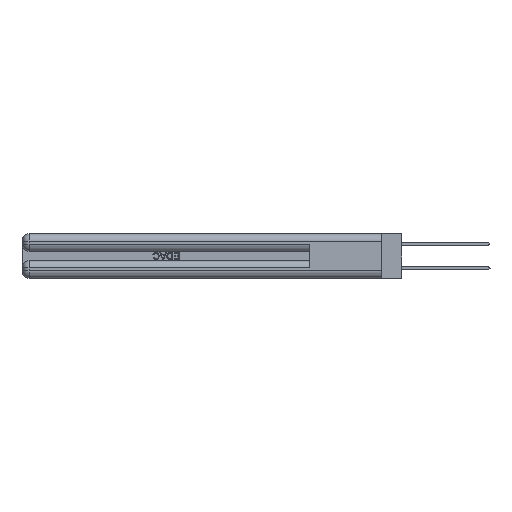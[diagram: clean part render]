
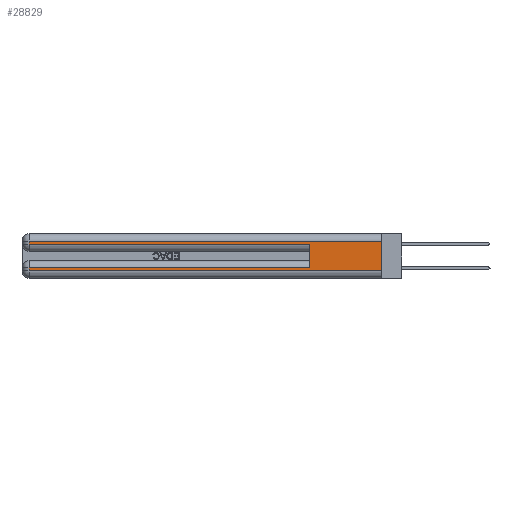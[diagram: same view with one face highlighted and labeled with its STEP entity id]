
A CAD part, left-side view. The second image highlights one B-rep face of the part: STEP entity #28829.
In plain terms, the highlighted planar face has unit normal (-1, 0, 0).
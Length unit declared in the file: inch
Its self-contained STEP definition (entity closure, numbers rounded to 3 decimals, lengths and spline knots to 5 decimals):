
#84 = EDGE_LOOP ( 'NONE', ( #25162, #44697, #18484, #17534, #12788, #21124, #45111, #26878 ) ) ;
#204 = LINE ( 'NONE', #20221, #9230 ) ;
#442 = CARTESIAN_POINT ( 'NONE',  ( 0., 2.94, 0.37 ) ) ;
#606 = LINE ( 'NONE', #25662, #39991 ) ;
#1106 = CARTESIAN_POINT ( 'NONE',  ( 0., 0., 0.285 ) ) ;
#1189 = DIRECTION ( 'NONE',  ( 0., -1., 0. ) ) ;
#2101 = DIRECTION ( 'NONE',  ( 0., 0., -1. ) ) ;
#2465 = LINE ( 'NONE', #12837, #32229 ) ;
#2803 = DIRECTION ( 'NONE',  ( 0., 0., -1. ) ) ;
#2838 = EDGE_CURVE ( 'NONE', #12835, #13054, #606, .T. ) ;
#3818 = AXIS2_PLACEMENT_3D ( 'NONE', #45466, #9768, #2101 ) ;
#4753 = DIRECTION ( 'NONE',  ( 0., -1., 0. ) ) ;
#5689 = VECTOR ( 'NONE', #1189, 39.37008 ) ;
#5760 = VERTEX_POINT ( 'NONE', #44814 ) ;
#6416 = DIRECTION ( 'NONE',  ( 0., 1., 0. ) ) ;
#9230 = VECTOR ( 'NONE', #2803, 39.37008 ) ;
#9733 = VECTOR ( 'NONE', #29216, 39.37008 ) ;
#9768 = DIRECTION ( 'NONE',  ( 1., 0., 0. ) ) ;
#10268 = EDGE_CURVE ( 'NONE', #5760, #13469, #204, .T. ) ;
#10463 = EDGE_CURVE ( 'NONE', #18079, #36989, #13769, .T. ) ;
#12788 = ORIENTED_EDGE ( 'NONE', *, *, #28244, .F. ) ;
#12835 = VERTEX_POINT ( 'NONE', #17748 ) ;
#12837 = CARTESIAN_POINT ( 'NONE',  ( 0., 0., 0.31 ) ) ;
#13054 = VERTEX_POINT ( 'NONE', #21293 ) ;
#13469 = VERTEX_POINT ( 'NONE', #37932 ) ;
#13769 = LINE ( 'NONE', #36397, #35679 ) ;
#14062 = LINE ( 'NONE', #40643, #5689 ) ;
#14242 = LINE ( 'NONE', #442, #9733 ) ;
#16396 = PLANE ( 'NONE',  #3818 ) ;
#16541 = EDGE_CURVE ( 'NONE', #13469, #19829, #45794, .T. ) ;
#16956 = EDGE_CURVE ( 'NONE', #18079, #5760, #2465, .T. ) ;
#17534 = ORIENTED_EDGE ( 'NONE', *, *, #16541, .T. ) ;
#17748 = CARTESIAN_POINT ( 'NONE',  ( 0., 0.6, 0.085 ) ) ;
#18079 = VERTEX_POINT ( 'NONE', #24294 ) ;
#18484 = ORIENTED_EDGE ( 'NONE', *, *, #10268, .T. ) ;
#19829 = VERTEX_POINT ( 'NONE', #42049 ) ;
#20221 = CARTESIAN_POINT ( 'NONE',  ( 0., 2.94, 0.37 ) ) ;
#21124 = ORIENTED_EDGE ( 'NONE', *, *, #2838, .T. ) ;
#21293 = CARTESIAN_POINT ( 'NONE',  ( 0., 2.94, 0.085 ) ) ;
#24294 = CARTESIAN_POINT ( 'NONE',  ( 0., 0., 0.31 ) ) ;
#24544 = EDGE_CURVE ( 'NONE', #13054, #43459, #14242, .T. ) ;
#25162 = ORIENTED_EDGE ( 'NONE', *, *, #10463, .F. ) ;
#25662 = CARTESIAN_POINT ( 'NONE',  ( 0., 0., 0.085 ) ) ;
#26263 = FACE_OUTER_BOUND ( 'NONE', #84, .T. ) ;
#26659 = VECTOR ( 'NONE', #4753, 39.37008 ) ;
#26878 = ORIENTED_EDGE ( 'NONE', *, *, #45808, .T. ) ;
#28244 = EDGE_CURVE ( 'NONE', #12835, #19829, #43758, .T. ) ;
#28829 = ADVANCED_FACE ( 'NONE', ( #26263 ), #16396, .F. ) ;
#29091 = CARTESIAN_POINT ( 'NONE',  ( 0., 2.94, 0.06 ) ) ;
#29216 = DIRECTION ( 'NONE',  ( 0., 0., -1. ) ) ;
#30127 = DIRECTION ( 'NONE',  ( 0., 0., 1. ) ) ;
#30285 = CARTESIAN_POINT ( 'NONE',  ( 0., 0.6, 0.145 ) ) ;
#30836 = VECTOR ( 'NONE', #30127, 39.37008 ) ;
#32229 = VECTOR ( 'NONE', #6416, 39.37008 ) ;
#35679 = VECTOR ( 'NONE', #36873, 39.37008 ) ;
#36397 = CARTESIAN_POINT ( 'NONE',  ( 0., 0., 0.37 ) ) ;
#36678 = CARTESIAN_POINT ( 'NONE',  ( 0., 0., 0.06 ) ) ;
#36873 = DIRECTION ( 'NONE',  ( 0., 0., -1. ) ) ;
#36989 = VERTEX_POINT ( 'NONE', #36678 ) ;
#37932 = CARTESIAN_POINT ( 'NONE',  ( 0., 2.94, 0.285 ) ) ;
#39991 = VECTOR ( 'NONE', #44232, 39.37008 ) ;
#40643 = CARTESIAN_POINT ( 'NONE',  ( 0., 0., 0.06 ) ) ;
#42049 = CARTESIAN_POINT ( 'NONE',  ( 0., 0.6, 0.285 ) ) ;
#43459 = VERTEX_POINT ( 'NONE', #29091 ) ;
#43758 = LINE ( 'NONE', #30285, #30836 ) ;
#44232 = DIRECTION ( 'NONE',  ( 0., 1., 0. ) ) ;
#44697 = ORIENTED_EDGE ( 'NONE', *, *, #16956, .T. ) ;
#44814 = CARTESIAN_POINT ( 'NONE',  ( 0., 2.94, 0.31 ) ) ;
#45111 = ORIENTED_EDGE ( 'NONE', *, *, #24544, .T. ) ;
#45466 = CARTESIAN_POINT ( 'NONE',  ( 0., 0., 0.37 ) ) ;
#45794 = LINE ( 'NONE', #1106, #26659 ) ;
#45808 = EDGE_CURVE ( 'NONE', #43459, #36989, #14062, .T. ) ;
